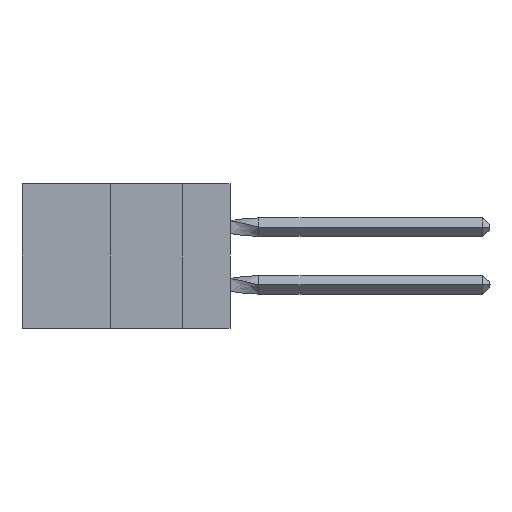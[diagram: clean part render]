
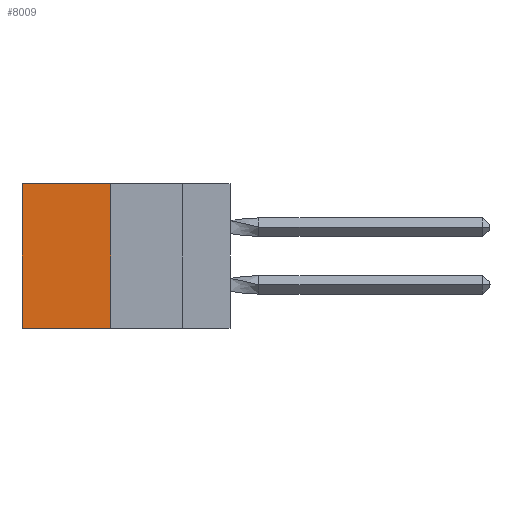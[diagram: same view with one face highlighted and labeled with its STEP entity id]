
A CAD part, left-side view. The second image highlights one B-rep face of the part: STEP entity #8009.
In plain terms, the highlighted planar face has unit normal (-1, 0, 0).
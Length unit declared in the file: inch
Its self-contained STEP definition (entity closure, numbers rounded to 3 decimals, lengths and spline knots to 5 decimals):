
#208 = VECTOR ( 'NONE', #3294, 39.37008 ) ;
#1668 = CARTESIAN_POINT ( 'NONE',  ( 0.305, 0.413, -0.5 ) ) ;
#2305 = DIRECTION ( 'NONE',  ( 0., 0., -1. ) ) ;
#2307 = LINE ( 'NONE', #6922, #7356 ) ;
#2903 = AXIS2_PLACEMENT_3D ( 'NONE', #1668, #5960, #4730 ) ;
#3294 = DIRECTION ( 'NONE',  ( 0., 0., -1. ) ) ;
#4319 = EDGE_CURVE ( 'NONE', #12582, #11957, #14686, .T. ) ;
#4397 = EDGE_LOOP ( 'NONE', ( #11415, #14757, #6950, #6324 ) ) ;
#4730 = DIRECTION ( 'NONE',  ( 0., 0., -1. ) ) ;
#5342 = FACE_OUTER_BOUND ( 'NONE', #4397, .T. ) ;
#5663 = DIRECTION ( 'NONE',  ( 0., 1., 0. ) ) ;
#5826 = CARTESIAN_POINT ( 'NONE',  ( 0.305, 0.72, 0. ) ) ;
#5893 = VECTOR ( 'NONE', #2305, 39.37008 ) ;
#5960 = DIRECTION ( 'NONE',  ( 1., 0., 0. ) ) ;
#6324 = ORIENTED_EDGE ( 'NONE', *, *, #15021, .T. ) ;
#6488 = EDGE_CURVE ( 'NONE', #10914, #12582, #7749, .T. ) ;
#6645 = CARTESIAN_POINT ( 'NONE',  ( 0.305, 0.413, -0.5 ) ) ;
#6922 = CARTESIAN_POINT ( 'NONE',  ( 0.305, 0.413, 0. ) ) ;
#6950 = ORIENTED_EDGE ( 'NONE', *, *, #6488, .F. ) ;
#7356 = VECTOR ( 'NONE', #11455, 39.37008 ) ;
#7654 = VECTOR ( 'NONE', #5663, 39.37008 ) ;
#7749 = LINE ( 'NONE', #18231, #5893 ) ;
#8009 = ADVANCED_FACE ( 'NONE', ( #5342 ), #14884, .F. ) ;
#9982 = CARTESIAN_POINT ( 'NONE',  ( 0.305, 0.72, -0.5 ) ) ;
#10914 = VERTEX_POINT ( 'NONE', #17984 ) ;
#11391 = LINE ( 'NONE', #11926, #208 ) ;
#11415 = ORIENTED_EDGE ( 'NONE', *, *, #11499, .T. ) ;
#11455 = DIRECTION ( 'NONE',  ( 0., 1., 0. ) ) ;
#11499 = EDGE_CURVE ( 'NONE', #17919, #11957, #11391, .T. ) ;
#11926 = CARTESIAN_POINT ( 'NONE',  ( 0.305, 0.72, -0.5 ) ) ;
#11957 = VERTEX_POINT ( 'NONE', #9982 ) ;
#12582 = VERTEX_POINT ( 'NONE', #6645 ) ;
#12884 = CARTESIAN_POINT ( 'NONE',  ( 0.305, 0.413, -0.5 ) ) ;
#14686 = LINE ( 'NONE', #12884, #7654 ) ;
#14757 = ORIENTED_EDGE ( 'NONE', *, *, #4319, .F. ) ;
#14884 = PLANE ( 'NONE',  #2903 ) ;
#15021 = EDGE_CURVE ( 'NONE', #10914, #17919, #2307, .T. ) ;
#17919 = VERTEX_POINT ( 'NONE', #5826 ) ;
#17984 = CARTESIAN_POINT ( 'NONE',  ( 0.305, 0.413, 0. ) ) ;
#18231 = CARTESIAN_POINT ( 'NONE',  ( 0.305, 0.413, -0.5 ) ) ;
